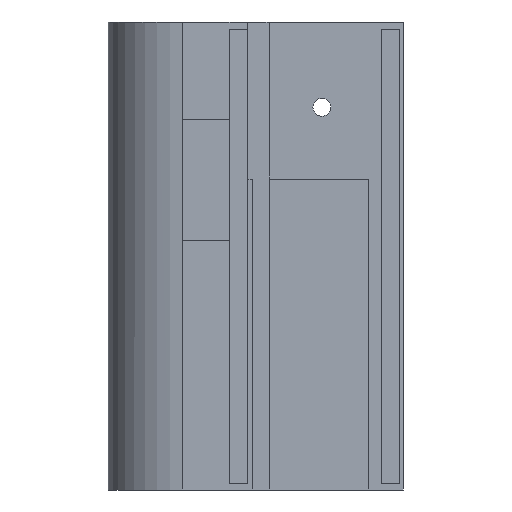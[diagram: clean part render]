
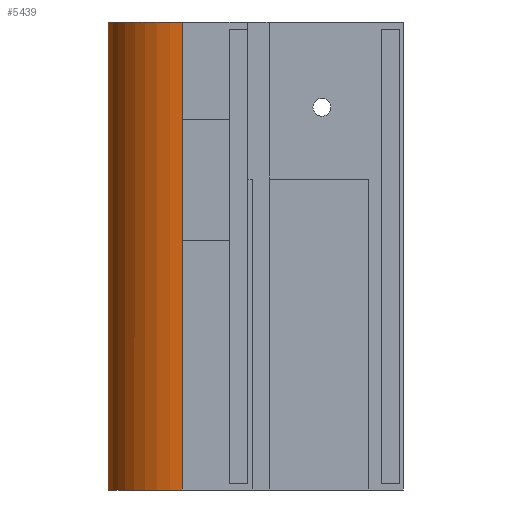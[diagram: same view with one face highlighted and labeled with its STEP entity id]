
A CAD part, left-side view. The second image highlights one B-rep face of the part: STEP entity #5439.
In plain terms, the highlighted cylindrical face has radius 13 mm (diameter 26 mm), a partial arc.
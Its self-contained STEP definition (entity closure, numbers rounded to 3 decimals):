
#1217 = PLANE('',#1218);
#1218 = AXIS2_PLACEMENT_3D('',#1219,#1220,#1221);
#1219 = CARTESIAN_POINT('',(-13.398,41.611,76.189));
#1220 = DIRECTION('',(0.,0.,1.));
#1221 = DIRECTION('',(1.,0.,0.));
#2781 = EDGE_CURVE('',#2782,#2784,#2786,.T.);
#2782 = VERTEX_POINT('',#2783);
#2783 = CARTESIAN_POINT('',(-12.982,25.692,76.189));
#2784 = VERTEX_POINT('',#2785);
#2785 = CARTESIAN_POINT('',(12.986,25.605,76.189));
#2786 = SURFACE_CURVE('',#2787,(#2792,#2803),.PCURVE_S1.);
#2787 = CIRCLE('',#2788,13.);
#2788 = AXIS2_PLACEMENT_3D('',#2789,#2790,#2791);
#2789 = CARTESIAN_POINT('',(0.,25.,76.189));
#2790 = DIRECTION('',(0.,0.,-1.));
#2791 = DIRECTION('',(1.,0.,0.));
#2792 = PCURVE('',#1217,#2793);
#2793 = DEFINITIONAL_REPRESENTATION('',(#2794),#2802);
#2794 = ( BOUNDED_CURVE() B_SPLINE_CURVE(2,(#2795,#2796,#2797,#2798,
#2799,#2800,#2801),.UNSPECIFIED.,.T.,.F.) B_SPLINE_CURVE_WITH_KNOTS((1,2
    ,2,2,2,1),(-2.094,0.,2.094,4.189,
6.283,8.378),.UNSPECIFIED.) CURVE() 
GEOMETRIC_REPRESENTATION_ITEM() RATIONAL_B_SPLINE_CURVE((1.,0.5,1.,0.5,
1.,0.5,1.)) REPRESENTATION_ITEM('') );
#2795 = CARTESIAN_POINT('',(26.398,-16.611));
#2796 = CARTESIAN_POINT('',(26.398,-39.127));
#2797 = CARTESIAN_POINT('',(6.898,-27.869));
#2798 = CARTESIAN_POINT('',(-12.602,-16.611));
#2799 = CARTESIAN_POINT('',(6.898,-5.352));
#2800 = CARTESIAN_POINT('',(26.398,5.906));
#2801 = CARTESIAN_POINT('',(26.398,-16.611));
#2802 = ( GEOMETRIC_REPRESENTATION_CONTEXT(2) 
PARAMETRIC_REPRESENTATION_CONTEXT() REPRESENTATION_CONTEXT('2D SPACE',''
  ) );
#2803 = PCURVE('',#2804,#2809);
#2804 = CYLINDRICAL_SURFACE('',#2805,13.);
#2805 = AXIS2_PLACEMENT_3D('',#2806,#2807,#2808);
#2806 = CARTESIAN_POINT('',(0.,25.,-1.));
#2807 = DIRECTION('',(0.,0.,-1.));
#2808 = DIRECTION('',(1.,0.,0.));
#2809 = DEFINITIONAL_REPRESENTATION('',(#2810),#2814);
#2810 = LINE('',#2811,#2812);
#2811 = CARTESIAN_POINT('',(0.,-77.189));
#2812 = VECTOR('',#2813,1.);
#2813 = DIRECTION('',(1.,0.));
#2814 = ( GEOMETRIC_REPRESENTATION_CONTEXT(2) 
PARAMETRIC_REPRESENTATION_CONTEXT() REPRESENTATION_CONTEXT('2D SPACE',''
  ) );
#2831 = PLANE('',#2832);
#2832 = AXIS2_PLACEMENT_3D('',#2833,#2834,#2835);
#2833 = CARTESIAN_POINT('',(-18.356,47.561,-1.));
#2834 = DIRECTION('',(0.971,0.239,0.));
#2835 = DIRECTION('',(0.239,-0.971,0.));
#3359 = PLANE('',#3360);
#3360 = AXIS2_PLACEMENT_3D('',#3361,#3362,#3363);
#3361 = CARTESIAN_POINT('',(12.986,25.605,-1.));
#3362 = DIRECTION('',(-0.989,0.145,0.));
#3363 = DIRECTION('',(0.145,0.989,0.));
#5439 = ADVANCED_FACE('',(#5440),#2804,.T.);
#5440 = FACE_BOUND('',#5441,.T.);
#5441 = EDGE_LOOP('',(#5442,#5473,#5494,#5495,#5518,#5547));
#5442 = ORIENTED_EDGE('',*,*,#5443,.F.);
#5443 = EDGE_CURVE('',#5444,#5446,#5448,.T.);
#5444 = VERTEX_POINT('',#5445);
#5445 = CARTESIAN_POINT('',(-12.982,25.692,-1.));
#5446 = VERTEX_POINT('',#5447);
#5447 = CARTESIAN_POINT('',(-11.,31.928,-1.));
#5448 = SURFACE_CURVE('',#5449,(#5454,#5461),.PCURVE_S1.);
#5449 = CIRCLE('',#5450,13.);
#5450 = AXIS2_PLACEMENT_3D('',#5451,#5452,#5453);
#5451 = CARTESIAN_POINT('',(0.,25.,-1.));
#5452 = DIRECTION('',(0.,0.,-1.));
#5453 = DIRECTION('',(1.,0.,0.));
#5454 = PCURVE('',#2804,#5455);
#5455 = DEFINITIONAL_REPRESENTATION('',(#5456),#5460);
#5456 = LINE('',#5457,#5458);
#5457 = CARTESIAN_POINT('',(0.,0.));
#5458 = VECTOR('',#5459,1.);
#5459 = DIRECTION('',(1.,0.));
#5460 = ( GEOMETRIC_REPRESENTATION_CONTEXT(2) 
PARAMETRIC_REPRESENTATION_CONTEXT() REPRESENTATION_CONTEXT('2D SPACE',''
  ) );
#5461 = PCURVE('',#5462,#5467);
#5462 = PLANE('',#5463);
#5463 = AXIS2_PLACEMENT_3D('',#5464,#5465,#5466);
#5464 = CARTESIAN_POINT('',(-13.,-5.,-1.));
#5465 = DIRECTION('',(0.,0.,-1.));
#5466 = DIRECTION('',(-1.,0.,0.));
#5467 = DEFINITIONAL_REPRESENTATION('',(#5468),#5472);
#5468 = CIRCLE('',#5469,13.);
#5469 = AXIS2_PLACEMENT_2D('',#5470,#5471);
#5470 = CARTESIAN_POINT('',(-13.,30.));
#5471 = DIRECTION('',(-1.,0.));
#5472 = ( GEOMETRIC_REPRESENTATION_CONTEXT(2) 
PARAMETRIC_REPRESENTATION_CONTEXT() REPRESENTATION_CONTEXT('2D SPACE',''
  ) );
#5473 = ORIENTED_EDGE('',*,*,#5474,.T.);
#5474 = EDGE_CURVE('',#5444,#2782,#5475,.T.);
#5475 = SURFACE_CURVE('',#5476,(#5480,#5487),.PCURVE_S1.);
#5476 = LINE('',#5477,#5478);
#5477 = CARTESIAN_POINT('',(-12.982,25.692,-1.));
#5478 = VECTOR('',#5479,1.);
#5479 = DIRECTION('',(0.,0.,1.));
#5480 = PCURVE('',#2804,#5481);
#5481 = DEFINITIONAL_REPRESENTATION('',(#5482),#5486);
#5482 = LINE('',#5483,#5484);
#5483 = CARTESIAN_POINT('',(3.195,0.));
#5484 = VECTOR('',#5485,1.);
#5485 = DIRECTION('',(0.,-1.));
#5486 = ( GEOMETRIC_REPRESENTATION_CONTEXT(2) 
PARAMETRIC_REPRESENTATION_CONTEXT() REPRESENTATION_CONTEXT('2D SPACE',''
  ) );
#5487 = PCURVE('',#2831,#5488);
#5488 = DEFINITIONAL_REPRESENTATION('',(#5489),#5493);
#5489 = LINE('',#5490,#5491);
#5490 = CARTESIAN_POINT('',(22.52,0.));
#5491 = VECTOR('',#5492,1.);
#5492 = DIRECTION('',(0.,-1.));
#5493 = ( GEOMETRIC_REPRESENTATION_CONTEXT(2) 
PARAMETRIC_REPRESENTATION_CONTEXT() REPRESENTATION_CONTEXT('2D SPACE',''
  ) );
#5494 = ORIENTED_EDGE('',*,*,#2781,.T.);
#5495 = ORIENTED_EDGE('',*,*,#5496,.F.);
#5496 = EDGE_CURVE('',#5497,#2784,#5499,.T.);
#5497 = VERTEX_POINT('',#5498);
#5498 = CARTESIAN_POINT('',(12.986,25.605,-1.));
#5499 = SURFACE_CURVE('',#5500,(#5504,#5511),.PCURVE_S1.);
#5500 = LINE('',#5501,#5502);
#5501 = CARTESIAN_POINT('',(12.986,25.605,-1.));
#5502 = VECTOR('',#5503,1.);
#5503 = DIRECTION('',(0.,0.,1.));
#5504 = PCURVE('',#2804,#5505);
#5505 = DEFINITIONAL_REPRESENTATION('',(#5506),#5510);
#5506 = LINE('',#5507,#5508);
#5507 = CARTESIAN_POINT('',(6.237,0.));
#5508 = VECTOR('',#5509,1.);
#5509 = DIRECTION('',(0.,-1.));
#5510 = ( GEOMETRIC_REPRESENTATION_CONTEXT(2) 
PARAMETRIC_REPRESENTATION_CONTEXT() REPRESENTATION_CONTEXT('2D SPACE',''
  ) );
#5511 = PCURVE('',#3359,#5512);
#5512 = DEFINITIONAL_REPRESENTATION('',(#5513),#5517);
#5513 = LINE('',#5514,#5515);
#5514 = CARTESIAN_POINT('',(0.,0.));
#5515 = VECTOR('',#5516,1.);
#5516 = DIRECTION('',(0.,-1.));
#5517 = ( GEOMETRIC_REPRESENTATION_CONTEXT(2) 
PARAMETRIC_REPRESENTATION_CONTEXT() REPRESENTATION_CONTEXT('2D SPACE',''
  ) );
#5518 = ORIENTED_EDGE('',*,*,#5519,.F.);
#5519 = EDGE_CURVE('',#5520,#5497,#5522,.T.);
#5520 = VERTEX_POINT('',#5521);
#5521 = CARTESIAN_POINT('',(11.,31.928,-1.));
#5522 = SURFACE_CURVE('',#5523,(#5528,#5535),.PCURVE_S1.);
#5523 = CIRCLE('',#5524,13.);
#5524 = AXIS2_PLACEMENT_3D('',#5525,#5526,#5527);
#5525 = CARTESIAN_POINT('',(0.,25.,-1.));
#5526 = DIRECTION('',(0.,0.,-1.));
#5527 = DIRECTION('',(1.,0.,0.));
#5528 = PCURVE('',#2804,#5529);
#5529 = DEFINITIONAL_REPRESENTATION('',(#5530),#5534);
#5530 = LINE('',#5531,#5532);
#5531 = CARTESIAN_POINT('',(0.,0.));
#5532 = VECTOR('',#5533,1.);
#5533 = DIRECTION('',(1.,0.));
#5534 = ( GEOMETRIC_REPRESENTATION_CONTEXT(2) 
PARAMETRIC_REPRESENTATION_CONTEXT() REPRESENTATION_CONTEXT('2D SPACE',''
  ) );
#5535 = PCURVE('',#5536,#5541);
#5536 = PLANE('',#5537);
#5537 = AXIS2_PLACEMENT_3D('',#5538,#5539,#5540);
#5538 = CARTESIAN_POINT('',(-13.,-5.,-1.));
#5539 = DIRECTION('',(0.,0.,-1.));
#5540 = DIRECTION('',(-1.,0.,0.));
#5541 = DEFINITIONAL_REPRESENTATION('',(#5542),#5546);
#5542 = CIRCLE('',#5543,13.);
#5543 = AXIS2_PLACEMENT_2D('',#5544,#5545);
#5544 = CARTESIAN_POINT('',(-13.,30.));
#5545 = DIRECTION('',(-1.,0.));
#5546 = ( GEOMETRIC_REPRESENTATION_CONTEXT(2) 
PARAMETRIC_REPRESENTATION_CONTEXT() REPRESENTATION_CONTEXT('2D SPACE',''
  ) );
#5547 = ORIENTED_EDGE('',*,*,#5548,.F.);
#5548 = EDGE_CURVE('',#5446,#5520,#5549,.T.);
#5549 = SURFACE_CURVE('',#5550,(#5555,#5562),.PCURVE_S1.);
#5550 = CIRCLE('',#5551,13.);
#5551 = AXIS2_PLACEMENT_3D('',#5552,#5553,#5554);
#5552 = CARTESIAN_POINT('',(0.,25.,-1.));
#5553 = DIRECTION('',(0.,0.,-1.));
#5554 = DIRECTION('',(1.,0.,0.));
#5555 = PCURVE('',#2804,#5556);
#5556 = DEFINITIONAL_REPRESENTATION('',(#5557),#5561);
#5557 = LINE('',#5558,#5559);
#5558 = CARTESIAN_POINT('',(0.,0.));
#5559 = VECTOR('',#5560,1.);
#5560 = DIRECTION('',(1.,0.));
#5561 = ( GEOMETRIC_REPRESENTATION_CONTEXT(2) 
PARAMETRIC_REPRESENTATION_CONTEXT() REPRESENTATION_CONTEXT('2D SPACE',''
  ) );
#5562 = PCURVE('',#5563,#5568);
#5563 = PLANE('',#5564);
#5564 = AXIS2_PLACEMENT_3D('',#5565,#5566,#5567);
#5565 = CARTESIAN_POINT('',(-13.,-5.,-1.));
#5566 = DIRECTION('',(0.,0.,-1.));
#5567 = DIRECTION('',(-1.,0.,0.));
#5568 = DEFINITIONAL_REPRESENTATION('',(#5569),#5573);
#5569 = CIRCLE('',#5570,13.);
#5570 = AXIS2_PLACEMENT_2D('',#5571,#5572);
#5571 = CARTESIAN_POINT('',(-13.,30.));
#5572 = DIRECTION('',(-1.,0.));
#5573 = ( GEOMETRIC_REPRESENTATION_CONTEXT(2) 
PARAMETRIC_REPRESENTATION_CONTEXT() REPRESENTATION_CONTEXT('2D SPACE',''
  ) );
